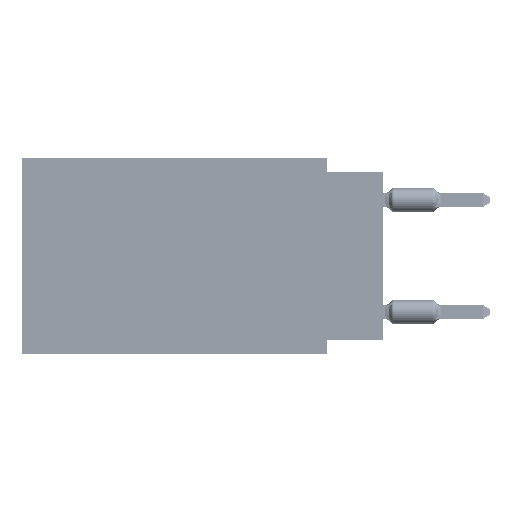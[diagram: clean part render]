
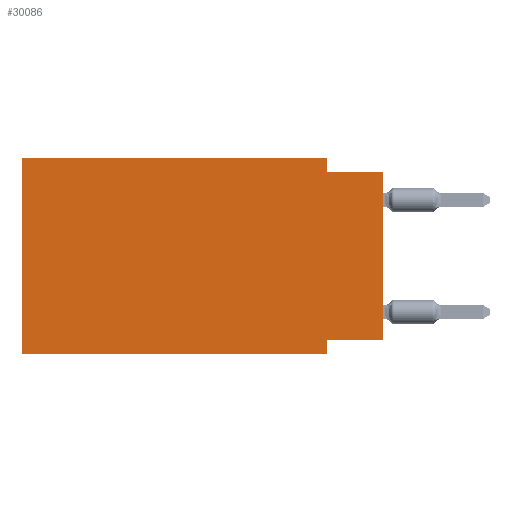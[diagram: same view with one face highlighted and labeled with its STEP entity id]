
A CAD part, left-side view. The second image highlights one B-rep face of the part: STEP entity #30086.
In plain terms, the highlighted planar face has unit normal (-1, 0, 0).
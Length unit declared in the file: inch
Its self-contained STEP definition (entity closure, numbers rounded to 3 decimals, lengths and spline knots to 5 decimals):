
#18 = ORIENTED_EDGE ( 'NONE', *, *, #56425, .T. ) ;
#295 = EDGE_CURVE ( 'NONE', #33895, #2070, #22170, .T. ) ;
#1452 = EDGE_CURVE ( 'NONE', #47572, #38970, #36560, .T. ) ;
#2037 = ORIENTED_EDGE ( 'NONE', *, *, #35287, .F. ) ;
#2070 = VERTEX_POINT ( 'NONE', #48683 ) ;
#2353 = DIRECTION ( 'NONE',  ( 0., -1., 0. ) ) ;
#7991 = VECTOR ( 'NONE', #2353, 39.37008 ) ;
#8825 = VECTOR ( 'NONE', #35865, 39.37008 ) ;
#8854 = DIRECTION ( 'NONE',  ( 0., 0., 1. ) ) ;
#8982 = LINE ( 'NONE', #67072, #7991 ) ;
#9882 = CARTESIAN_POINT ( 'NONE',  ( 0., 0., 0. ) ) ;
#10247 = LINE ( 'NONE', #58511, #16179 ) ;
#13123 = DIRECTION ( 'NONE',  ( 1., 0., 0. ) ) ;
#16179 = VECTOR ( 'NONE', #26385, 39.37008 ) ;
#18630 = ORIENTED_EDGE ( 'NONE', *, *, #38995, .F. ) ;
#20795 = AXIS2_PLACEMENT_3D ( 'NONE', #61036, #13123, #50541 ) ;
#22170 = LINE ( 'NONE', #43519, #36677 ) ;
#22988 = EDGE_CURVE ( 'NONE', #2070, #44339, #23401, .T. ) ;
#23048 = ORIENTED_EDGE ( 'NONE', *, *, #66455, .T. ) ;
#23401 = LINE ( 'NONE', #49622, #30803 ) ;
#25984 = EDGE_LOOP ( 'NONE', ( #18, #68905, #28382, #2037, #43586, #23048, #26369, #18630 ) ) ;
#26369 = ORIENTED_EDGE ( 'NONE', *, *, #1452, .F. ) ;
#26385 = DIRECTION ( 'NONE',  ( 0., -1., 0. ) ) ;
#27871 = VERTEX_POINT ( 'NONE', #65042 ) ;
#28382 = ORIENTED_EDGE ( 'NONE', *, *, #295, .F. ) ;
#30086 = ADVANCED_FACE ( 'NONE', ( #50220 ), #39738, .F. ) ;
#30803 = VECTOR ( 'NONE', #38816, 39.37008 ) ;
#32709 = CARTESIAN_POINT ( 'NONE',  ( 0., 0.1, -0.35 ) ) ;
#33895 = VERTEX_POINT ( 'NONE', #59424 ) ;
#35287 = EDGE_CURVE ( 'NONE', #27871, #33895, #8982, .T. ) ;
#35865 = DIRECTION ( 'NONE',  ( 0., 0., -1. ) ) ;
#36560 = LINE ( 'NONE', #47049, #8825 ) ;
#36677 = VECTOR ( 'NONE', #47730, 39.37008 ) ;
#37629 = DIRECTION ( 'NONE',  ( 0., 1., 0. ) ) ;
#37723 = CARTESIAN_POINT ( 'NONE',  ( 0., 0.645, 0. ) ) ;
#38816 = DIRECTION ( 'NONE',  ( 0., -1., 0. ) ) ;
#38970 = VERTEX_POINT ( 'NONE', #32709 ) ;
#38995 = EDGE_CURVE ( 'NONE', #63858, #47572, #49489, .T. ) ;
#39738 = PLANE ( 'NONE',  #20795 ) ;
#43519 = CARTESIAN_POINT ( 'NONE',  ( 0., 0.1, 0. ) ) ;
#43586 = ORIENTED_EDGE ( 'NONE', *, *, #47804, .F. ) ;
#44339 = VERTEX_POINT ( 'NONE', #62388 ) ;
#46181 = VERTEX_POINT ( 'NONE', #60496 ) ;
#46303 = LINE ( 'NONE', #9882, #65618 ) ;
#47049 = CARTESIAN_POINT ( 'NONE',  ( 0., 0.1, -0.35 ) ) ;
#47461 = VECTOR ( 'NONE', #37629, 39.37008 ) ;
#47572 = VERTEX_POINT ( 'NONE', #67132 ) ;
#47730 = DIRECTION ( 'NONE',  ( 0., 0., -1. ) ) ;
#47804 = EDGE_CURVE ( 'NONE', #46181, #27871, #48205, .T. ) ;
#48205 = LINE ( 'NONE', #37723, #49201 ) ;
#48683 = CARTESIAN_POINT ( 'NONE',  ( 0., 0.1, -0.025 ) ) ;
#48821 = CARTESIAN_POINT ( 'NONE',  ( 0., 0., -0.325 ) ) ;
#49201 = VECTOR ( 'NONE', #64262, 39.37008 ) ;
#49489 = LINE ( 'NONE', #48821, #47461 ) ;
#49622 = CARTESIAN_POINT ( 'NONE',  ( 0., 0., -0.025 ) ) ;
#50220 = FACE_OUTER_BOUND ( 'NONE', #25984, .T. ) ;
#50541 = DIRECTION ( 'NONE',  ( 0., 0., -1. ) ) ;
#56425 = EDGE_CURVE ( 'NONE', #63858, #44339, #46303, .T. ) ;
#58511 = CARTESIAN_POINT ( 'NONE',  ( 0., 0.645, -0.35 ) ) ;
#59424 = CARTESIAN_POINT ( 'NONE',  ( 0., 0.1, 0. ) ) ;
#60496 = CARTESIAN_POINT ( 'NONE',  ( 0., 0.645, -0.35 ) ) ;
#61036 = CARTESIAN_POINT ( 'NONE',  ( 0., 0.645, 0. ) ) ;
#61579 = CARTESIAN_POINT ( 'NONE',  ( 0., 0., -0.325 ) ) ;
#62388 = CARTESIAN_POINT ( 'NONE',  ( 0., 0., -0.025 ) ) ;
#63858 = VERTEX_POINT ( 'NONE', #61579 ) ;
#64262 = DIRECTION ( 'NONE',  ( 0., 0., 1. ) ) ;
#65042 = CARTESIAN_POINT ( 'NONE',  ( 0., 0.645, 0. ) ) ;
#65618 = VECTOR ( 'NONE', #8854, 39.37008 ) ;
#66455 = EDGE_CURVE ( 'NONE', #46181, #38970, #10247, .T. ) ;
#67072 = CARTESIAN_POINT ( 'NONE',  ( 0., 0.645, 0. ) ) ;
#67132 = CARTESIAN_POINT ( 'NONE',  ( 0., 0.1, -0.325 ) ) ;
#68905 = ORIENTED_EDGE ( 'NONE', *, *, #22988, .F. ) ;
